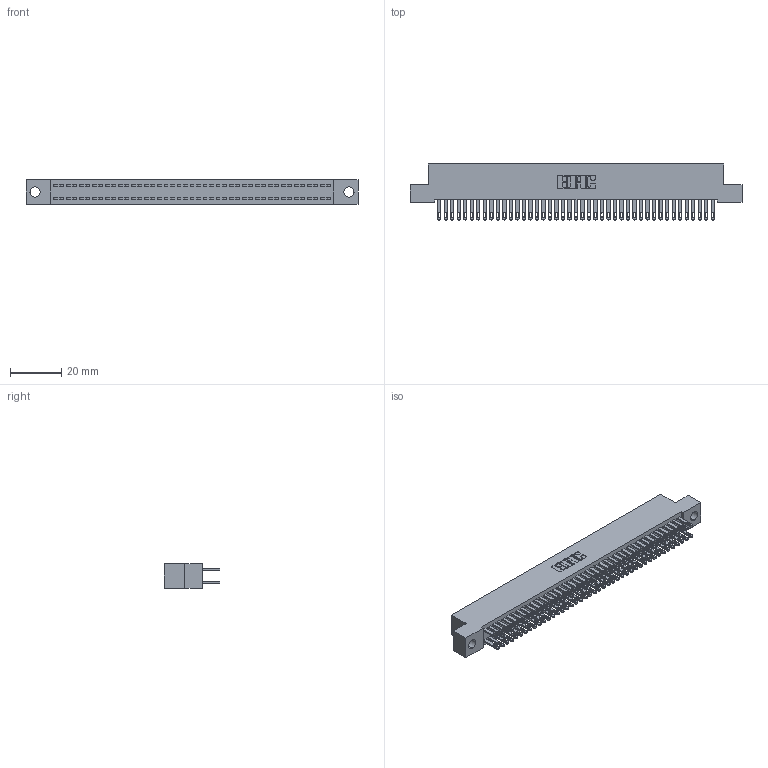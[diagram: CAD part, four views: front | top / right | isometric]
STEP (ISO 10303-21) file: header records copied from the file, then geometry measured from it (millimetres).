
FILE_DESCRIPTION (( 'STEP AP203' ), '1' );
FILE_NAME ('892-086-500-204.STEP', '2020-09-21T20:31:45', ( '' ), ( '' ), 'SwSTEP 2.0', 'SolidWorks 2020', '' );
FILE_SCHEMA (( 'CONFIG_CONTROL_DESIGN' ));
Length unit declared in the file: inch
Products named in the file (3): 842 Part_.156 TH; 892-086-500-204; 345-292-001_345-293-100
Assembly tree (87 placements, depth 2):
  892-086-500-204
    842 Part_.156 TH
    345-292-001_345-293-100  x86
Bounding box: 129.54 x 21.85 x 9.4 mm (x, y, z)
Volume: 11819.7 mm3; surface area: 19911.7 mm2
Topology: 87 solids, 87 shells, 4238 faces, 12941 edges, 8626 vertices
Faces by surface type: plane 2646, cylinder 1592
Entity records: 27335 total; most frequent: CARTESIAN_POINT 4526, ORIENTED_EDGE 4462, DIRECTION 3867, EDGE_CURVE 2231, VECTOR 2099, LINE 2099, VERTEX_POINT 1486, AXIS2_PLACEMENT_3D 884
